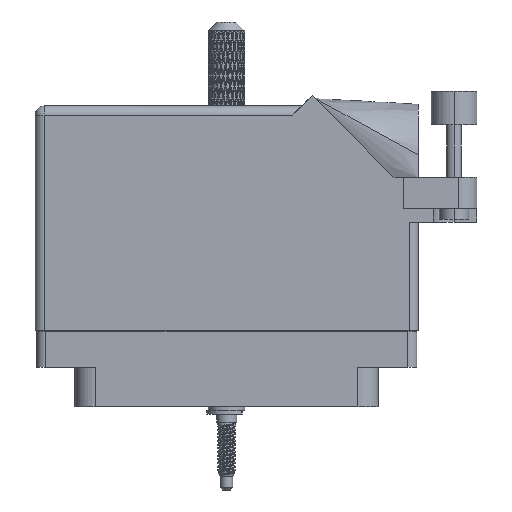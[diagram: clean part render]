
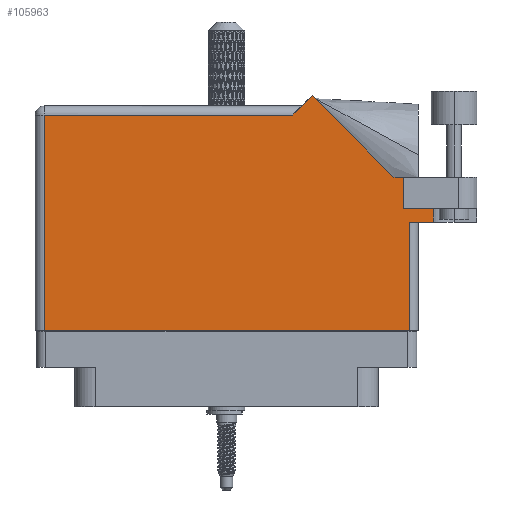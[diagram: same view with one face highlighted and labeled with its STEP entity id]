
A CAD part, front view. The second image highlights one B-rep face of the part: STEP entity #105963.
In plain terms, the highlighted face is planar.
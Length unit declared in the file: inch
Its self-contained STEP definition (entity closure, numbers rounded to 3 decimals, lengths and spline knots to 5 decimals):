
#3563 = VECTOR ( 'NONE', #68836, 39.37008 ) ;
#4117 = VECTOR ( 'NONE', #57129, 39.37008 ) ;
#4625 = VECTOR ( 'NONE', #99861, 39.37008 ) ;
#4872 = DIRECTION ( 'NONE',  ( -1., 0., 0. ) ) ;
#5393 = VERTEX_POINT ( 'NONE', #29759 ) ;
#6356 = VERTEX_POINT ( 'NONE', #98042 ) ;
#7224 = CARTESIAN_POINT ( 'NONE',  ( 1.244, 0.637, 0.455 ) ) ;
#8037 = CARTESIAN_POINT ( 'NONE',  ( -1.244, -0.1, 0.455 ) ) ;
#8452 = EDGE_CURVE ( 'NONE', #86511, #85837, #28883, .T. ) ;
#10361 = LINE ( 'NONE', #98905, #80252 ) ;
#10363 = EDGE_CURVE ( 'NONE', #6356, #86511, #29915, .T. ) ;
#10391 = ORIENTED_EDGE ( 'NONE', *, *, #84256, .T. ) ;
#11388 = ORIENTED_EDGE ( 'NONE', *, *, #46973, .F. ) ;
#12835 = ORIENTED_EDGE ( 'NONE', *, *, #30666, .T. ) ;
#13184 = EDGE_CURVE ( 'NONE', #64778, #6356, #116090, .T. ) ;
#13363 = VECTOR ( 'NONE', #16024, 39.37008 ) ;
#14797 = EDGE_CURVE ( 'NONE', #68533, #64778, #10361, .T. ) ;
#16024 = DIRECTION ( 'NONE',  ( 0., 1., 0. ) ) ;
#19810 = LINE ( 'NONE', #52050, #34275 ) ;
#21240 = EDGE_CURVE ( 'NONE', #65910, #58199, #83588, .T. ) ;
#24494 = CARTESIAN_POINT ( 'NONE',  ( 1.706, 0.944, 0.455 ) ) ;
#24993 = CARTESIAN_POINT ( 'NONE',  ( 1.306, 0.637, 0.455 ) ) ;
#26647 = VERTEX_POINT ( 'NONE', #38618 ) ;
#27256 = VERTEX_POINT ( 'NONE', #64008 ) ;
#28038 = CARTESIAN_POINT ( 'NONE',  ( 1.206, 0.731, 0.455 ) ) ;
#28883 = LINE ( 'NONE', #36228, #4625 ) ;
#29759 = CARTESIAN_POINT ( 'NONE',  ( 1.4075, 0.731, 0.455 ) ) ;
#29915 = LINE ( 'NONE', #58340, #38556 ) ;
#30449 = CARTESIAN_POINT ( 'NONE',  ( 1.206, 0.944, 0.455 ) ) ;
#30666 = EDGE_CURVE ( 'NONE', #58199, #27256, #94885, .T. ) ;
#32137 = VERTEX_POINT ( 'NONE', #7224 ) ;
#32906 = PLANE ( 'NONE',  #39858 ) ;
#34275 = VECTOR ( 'NONE', #69963, 39.37008 ) ;
#36228 = CARTESIAN_POINT ( 'NONE',  ( 0.513, 1.43, 0.455 ) ) ;
#38556 = VECTOR ( 'NONE', #67562, 39.37008 ) ;
#38618 = CARTESIAN_POINT ( 'NONE',  ( 1.4075, 0.637, 0.455 ) ) ;
#38848 = ORIENTED_EDGE ( 'NONE', *, *, #80956, .F. ) ;
#39858 = AXIS2_PLACEMENT_3D ( 'NONE', #116009, #52025, #42831 ) ;
#42289 = VECTOR ( 'NONE', #70283, 39.37008 ) ;
#42831 = DIRECTION ( 'NONE',  ( -1., 0., 0. ) ) ;
#42912 = EDGE_LOOP ( 'NONE', ( #12835, #101782, #10391, #38848, #11388, #76694, #70083, #45504, #98162, #75017, #70177 ) ) ;
#44539 = LINE ( 'NONE', #58695, #81487 ) ;
#44878 = CARTESIAN_POINT ( 'NONE',  ( -1.244, 1.368, 0.455 ) ) ;
#45504 = ORIENTED_EDGE ( 'NONE', *, *, #10363, .T. ) ;
#46973 = EDGE_CURVE ( 'NONE', #68533, #5393, #106736, .T. ) ;
#47672 = CARTESIAN_POINT ( 'NONE',  ( -1.306, -0.1, 0.455 ) ) ;
#48049 = DIRECTION ( 'NONE',  ( 1., 0., 0. ) ) ;
#52025 = DIRECTION ( 'NONE',  ( 0., 0., -1. ) ) ;
#52050 = CARTESIAN_POINT ( 'NONE',  ( 1.4075, 1.06177, 0.455 ) ) ;
#53400 = LINE ( 'NONE', #60776, #13363 ) ;
#57129 = DIRECTION ( 'NONE',  ( 1., 0., 0. ) ) ;
#58199 = VERTEX_POINT ( 'NONE', #84852 ) ;
#58340 = CARTESIAN_POINT ( 'NONE',  ( 1.14042, 0.944, 0.455 ) ) ;
#58695 = CARTESIAN_POINT ( 'NONE',  ( -1.306, 1.368, 0.455 ) ) ;
#60776 = CARTESIAN_POINT ( 'NONE',  ( 1.244, 0.637, 0.455 ) ) ;
#62082 = CARTESIAN_POINT ( 'NONE',  ( 1.206, 0.731, 0.455 ) ) ;
#64008 = CARTESIAN_POINT ( 'NONE',  ( 1.244, -0.1, 0.455 ) ) ;
#64778 = VERTEX_POINT ( 'NONE', #30449 ) ;
#65910 = VERTEX_POINT ( 'NONE', #44878 ) ;
#67562 = DIRECTION ( 'NONE',  ( -0.707, 0.707, 0. ) ) ;
#68533 = VERTEX_POINT ( 'NONE', #62082 ) ;
#68836 = DIRECTION ( 'NONE',  ( -1., 0., 0. ) ) ;
#68891 = FACE_OUTER_BOUND ( 'NONE', #42912, .T. ) ;
#69963 = DIRECTION ( 'NONE',  ( 0., -1., 0. ) ) ;
#70083 = ORIENTED_EDGE ( 'NONE', *, *, #13184, .T. ) ;
#70177 = ORIENTED_EDGE ( 'NONE', *, *, #21240, .T. ) ;
#70283 = DIRECTION ( 'NONE',  ( 0., -1., 0. ) ) ;
#75017 = ORIENTED_EDGE ( 'NONE', *, *, #79010, .T. ) ;
#76694 = ORIENTED_EDGE ( 'NONE', *, *, #14797, .T. ) ;
#79010 = EDGE_CURVE ( 'NONE', #85837, #65910, #44539, .T. ) ;
#80252 = VECTOR ( 'NONE', #89313, 39.37008 ) ;
#80956 = EDGE_CURVE ( 'NONE', #5393, #26647, #19810, .T. ) ;
#81487 = VECTOR ( 'NONE', #4872, 39.37008 ) ;
#82537 = CARTESIAN_POINT ( 'NONE',  ( 0.451, 1.368, 0.455 ) ) ;
#83588 = LINE ( 'NONE', #8037, #42289 ) ;
#84256 = EDGE_CURVE ( 'NONE', #32137, #26647, #97101, .T. ) ;
#84852 = CARTESIAN_POINT ( 'NONE',  ( -1.244, -0.1, 0.455 ) ) ;
#85837 = VERTEX_POINT ( 'NONE', #82537 ) ;
#86511 = VERTEX_POINT ( 'NONE', #96961 ) ;
#89313 = DIRECTION ( 'NONE',  ( 0., 1., 0. ) ) ;
#94885 = LINE ( 'NONE', #47672, #104757 ) ;
#96961 = CARTESIAN_POINT ( 'NONE',  ( 0.58371, 1.50071, 0.455 ) ) ;
#97101 = LINE ( 'NONE', #24993, #112644 ) ;
#98042 = CARTESIAN_POINT ( 'NONE',  ( 1.14042, 0.944, 0.455 ) ) ;
#98162 = ORIENTED_EDGE ( 'NONE', *, *, #8452, .T. ) ;
#98905 = CARTESIAN_POINT ( 'NONE',  ( 1.206, 0.731, 0.455 ) ) ;
#99861 = DIRECTION ( 'NONE',  ( -0.707, -0.707, 0. ) ) ;
#101782 = ORIENTED_EDGE ( 'NONE', *, *, #103157, .T. ) ;
#103157 = EDGE_CURVE ( 'NONE', #27256, #32137, #53400, .T. ) ;
#104757 = VECTOR ( 'NONE', #48049, 39.37008 ) ;
#105963 = ADVANCED_FACE ( 'NONE', ( #68891 ), #32906, .F. ) ;
#106736 = LINE ( 'NONE', #28038, #4117 ) ;
#112644 = VECTOR ( 'NONE', #117699, 39.37008 ) ;
#116009 = CARTESIAN_POINT ( 'NONE',  ( -1.306, 1.43, 0.455 ) ) ;
#116090 = LINE ( 'NONE', #24494, #3563 ) ;
#117699 = DIRECTION ( 'NONE',  ( 1., 0., 0. ) ) ;
